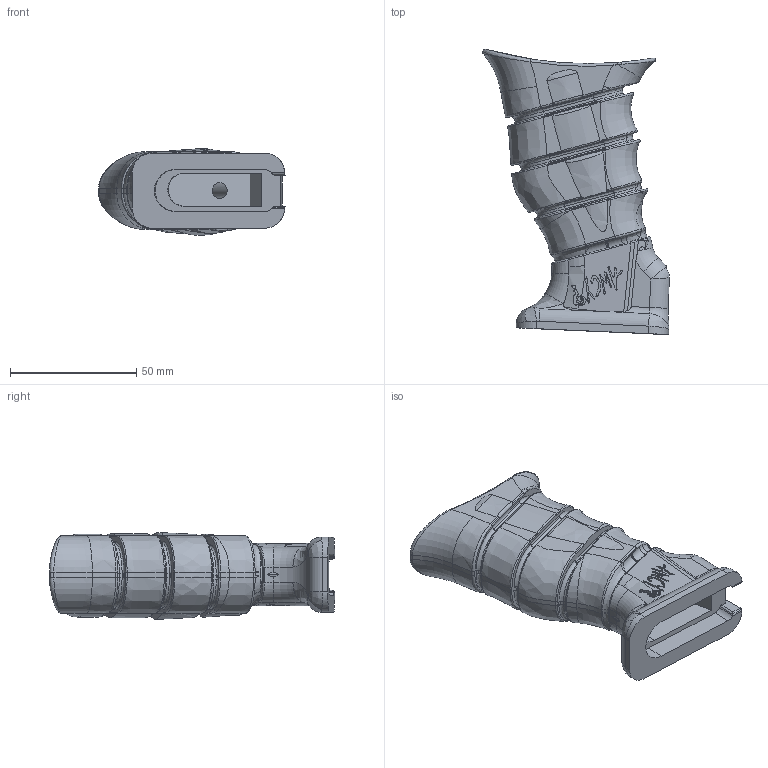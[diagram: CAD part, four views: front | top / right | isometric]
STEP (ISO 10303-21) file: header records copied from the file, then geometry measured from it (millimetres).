
FILE_DESCRIPTION(('STEP AP214'),'1');
FILE_NAME('AKaBargrip Final.stp','2021-07-22T20:39:01',(' '),(' '),'Spatial InterOp 3D',' ',' ');
FILE_SCHEMA(('AUTOMOTIVE_DESIGN { 1 0 10303 214 1 1 1 1 }'));
Length unit declared in the file: metre
Products named in the file (3): revised kabar grip full assembly boke; revised kabar grip full assembly; AKaBargrip Final
Assembly tree (2 placements, depth 3):
  AKaBargrip Final
    revised kabar grip full assembly boke
      revised kabar grip full assembly
Bounding box: 73.86 x 112.78 x 34.35 mm (x, y, z)
Volume: 121287.1 mm3; surface area: 27458.6 mm2
Topology: 1 solids, 1 shells, 961 faces, 2604 edges, 1659 vertices
Faces by surface type: plane 260, bspline 228, extrusion 222, cylinder 220, torus 31
Entity records: 102335 total; most frequent: CARTESIAN_POINT 80414, ORIENTED_EDGE 5190, DIRECTION 3400, EDGE_CURVE 2595, VERTEX_POINT 1657, VECTOR 1262, B_SPLINE_CURVE_WITH_KNOTS 1222, AXIS2_PLACEMENT_3D 1069
